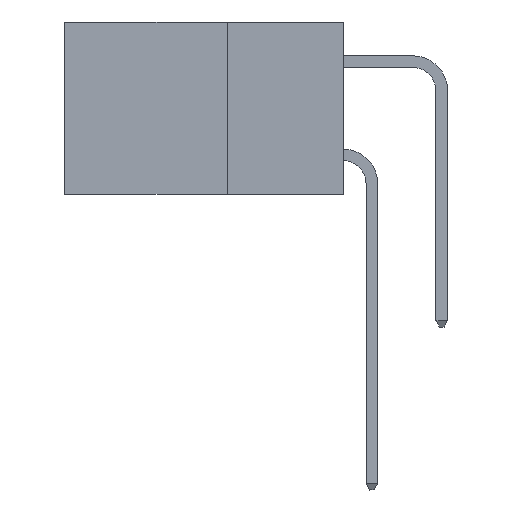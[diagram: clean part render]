
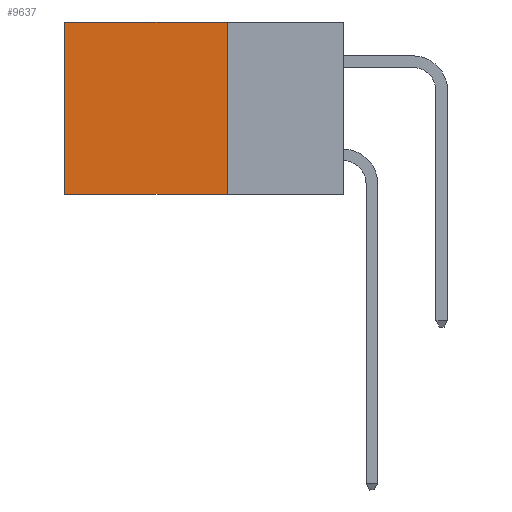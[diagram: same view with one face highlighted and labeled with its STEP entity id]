
A CAD part, left-side view. The second image highlights one B-rep face of the part: STEP entity #9637.
In plain terms, the highlighted planar face has unit normal (-1, 0, 0).
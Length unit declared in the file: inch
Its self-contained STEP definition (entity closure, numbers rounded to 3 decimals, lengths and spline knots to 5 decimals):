
#26 = FACE_OUTER_BOUND ( 'NONE', #13221, .T. ) ;
#63 = VECTOR ( 'NONE', #4223, 39.37008 ) ;
#66 = CARTESIAN_POINT ( 'NONE',  ( 0.2615, 0.25, -0.37 ) ) ;
#1234 = VECTOR ( 'NONE', #15882, 39.37008 ) ;
#1306 = EDGE_CURVE ( 'NONE', #17223, #1758, #15147, .T. ) ;
#1758 = VERTEX_POINT ( 'NONE', #22682 ) ;
#1853 = LINE ( 'NONE', #13950, #1234 ) ;
#2063 = DIRECTION ( 'NONE',  ( 0., 0., -1. ) ) ;
#3701 = CARTESIAN_POINT ( 'NONE',  ( 0.2615, 0.25, 0. ) ) ;
#3938 = CARTESIAN_POINT ( 'NONE',  ( 0.2615, 0.25, 0. ) ) ;
#4223 = DIRECTION ( 'NONE',  ( 0., 1., 0. ) ) ;
#4983 = LINE ( 'NONE', #6301, #25047 ) ;
#5184 = DIRECTION ( 'NONE',  ( 0., 1., 0. ) ) ;
#5741 = EDGE_CURVE ( 'NONE', #17223, #23248, #1853, .T. ) ;
#5817 = EDGE_CURVE ( 'NONE', #1758, #25199, #4983, .T. ) ;
#6301 = CARTESIAN_POINT ( 'NONE',  ( 0.2615, 0.6, -0.37 ) ) ;
#7353 = EDGE_CURVE ( 'NONE', #23248, #25199, #11093, .T. ) ;
#9637 = ADVANCED_FACE ( 'NONE', ( #26 ), #11905, .F. ) ;
#9911 = AXIS2_PLACEMENT_3D ( 'NONE', #66, #13855, #2063 ) ;
#10330 = ORIENTED_EDGE ( 'NONE', *, *, #7353, .F. ) ;
#10652 = ORIENTED_EDGE ( 'NONE', *, *, #5817, .T. ) ;
#11093 = LINE ( 'NONE', #13002, #15638 ) ;
#11905 = PLANE ( 'NONE',  #9911 ) ;
#12231 = DIRECTION ( 'NONE',  ( 0., 0., -1. ) ) ;
#13002 = CARTESIAN_POINT ( 'NONE',  ( 0.2615, 0.25, -0.37 ) ) ;
#13221 = EDGE_LOOP ( 'NONE', ( #10652, #10330, #19065, #23582 ) ) ;
#13855 = DIRECTION ( 'NONE',  ( 1., 0., 0. ) ) ;
#13950 = CARTESIAN_POINT ( 'NONE',  ( 0.2615, 0.25, -0.37 ) ) ;
#15147 = LINE ( 'NONE', #3938, #63 ) ;
#15638 = VECTOR ( 'NONE', #5184, 39.37008 ) ;
#15882 = DIRECTION ( 'NONE',  ( 0., 0., -1. ) ) ;
#15972 = CARTESIAN_POINT ( 'NONE',  ( 0.2615, 0.25, -0.37 ) ) ;
#17223 = VERTEX_POINT ( 'NONE', #3701 ) ;
#18091 = CARTESIAN_POINT ( 'NONE',  ( 0.2615, 0.6, -0.37 ) ) ;
#19065 = ORIENTED_EDGE ( 'NONE', *, *, #5741, .F. ) ;
#22682 = CARTESIAN_POINT ( 'NONE',  ( 0.2615, 0.6, 0. ) ) ;
#23248 = VERTEX_POINT ( 'NONE', #15972 ) ;
#23582 = ORIENTED_EDGE ( 'NONE', *, *, #1306, .T. ) ;
#25047 = VECTOR ( 'NONE', #12231, 39.37008 ) ;
#25199 = VERTEX_POINT ( 'NONE', #18091 ) ;
